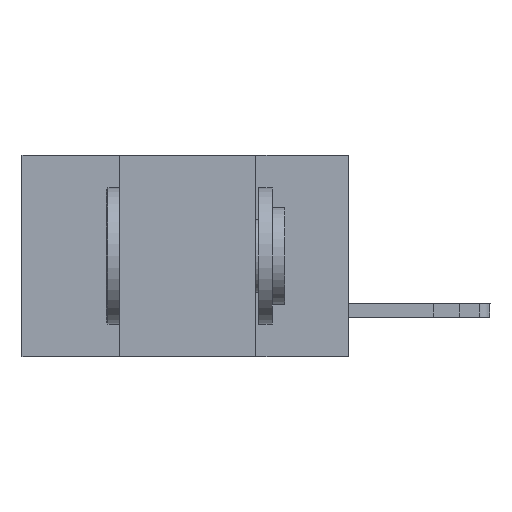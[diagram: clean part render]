
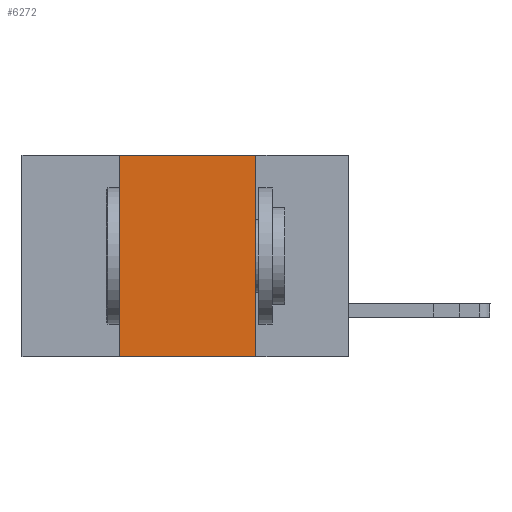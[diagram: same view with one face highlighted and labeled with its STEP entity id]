
A CAD part, left-side view. The second image highlights one B-rep face of the part: STEP entity #6272.
In plain terms, the highlighted planar face has unit normal (-1, 0, 0).
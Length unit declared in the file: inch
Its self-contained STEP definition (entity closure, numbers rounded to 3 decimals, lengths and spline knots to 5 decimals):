
#398 = VERTEX_POINT ( 'NONE', #16084 ) ;
#685 = ORIENTED_EDGE ( 'NONE', *, *, #16690, .F. ) ;
#1349 = EDGE_CURVE ( 'NONE', #14114, #12166, #11233, .T. ) ;
#2621 = CARTESIAN_POINT ( 'NONE',  ( 0., 0.42, -0.37 ) ) ;
#2738 = VECTOR ( 'NONE', #12178, 39.37008 ) ;
#2778 = CARTESIAN_POINT ( 'NONE',  ( 0., 0.6, -0.37 ) ) ;
#3225 = ORIENTED_EDGE ( 'NONE', *, *, #12811, .T. ) ;
#3415 = DIRECTION ( 'NONE',  ( 1., 0., 0. ) ) ;
#4107 = VERTEX_POINT ( 'NONE', #16202 ) ;
#4130 = DIRECTION ( 'NONE',  ( 0., 0., 1. ) ) ;
#5352 = LINE ( 'NONE', #6187, #16735 ) ;
#6187 = CARTESIAN_POINT ( 'NONE',  ( 0., 0.6, 0. ) ) ;
#6272 = ADVANCED_FACE ( 'NONE', ( #17154 ), #11888, .F. ) ;
#6337 = VECTOR ( 'NONE', #4130, 39.37008 ) ;
#6991 = CARTESIAN_POINT ( 'NONE',  ( 0., 0.6, 0. ) ) ;
#7690 = DIRECTION ( 'NONE',  ( 0., 0., -1. ) ) ;
#7740 = AXIS2_PLACEMENT_3D ( 'NONE', #6991, #3415, #7690 ) ;
#9054 = EDGE_LOOP ( 'NONE', ( #10799, #685, #9604, #3225 ) ) ;
#9604 = ORIENTED_EDGE ( 'NONE', *, *, #15727, .F. ) ;
#10799 = ORIENTED_EDGE ( 'NONE', *, *, #1349, .F. ) ;
#11233 = LINE ( 'NONE', #11684, #2738 ) ;
#11528 = LINE ( 'NONE', #2778, #12010 ) ;
#11684 = CARTESIAN_POINT ( 'NONE',  ( 0., 0.17, -0.37 ) ) ;
#11888 = PLANE ( 'NONE',  #7740 ) ;
#12010 = VECTOR ( 'NONE', #14726, 39.37008 ) ;
#12166 = VERTEX_POINT ( 'NONE', #18737 ) ;
#12178 = DIRECTION ( 'NONE',  ( 0., 0., -1. ) ) ;
#12665 = CARTESIAN_POINT ( 'NONE',  ( 0., 0.17, 0. ) ) ;
#12811 = EDGE_CURVE ( 'NONE', #4107, #12166, #11528, .T. ) ;
#14114 = VERTEX_POINT ( 'NONE', #12665 ) ;
#14726 = DIRECTION ( 'NONE',  ( 0., -1., 0. ) ) ;
#15727 = EDGE_CURVE ( 'NONE', #4107, #398, #18097, .T. ) ;
#16084 = CARTESIAN_POINT ( 'NONE',  ( 0., 0.42, 0. ) ) ;
#16202 = CARTESIAN_POINT ( 'NONE',  ( 0., 0.42, -0.37 ) ) ;
#16690 = EDGE_CURVE ( 'NONE', #398, #14114, #5352, .T. ) ;
#16735 = VECTOR ( 'NONE', #18805, 39.37008 ) ;
#17154 = FACE_OUTER_BOUND ( 'NONE', #9054, .T. ) ;
#18097 = LINE ( 'NONE', #2621, #6337 ) ;
#18737 = CARTESIAN_POINT ( 'NONE',  ( 0., 0.17, -0.37 ) ) ;
#18805 = DIRECTION ( 'NONE',  ( 0., -1., 0. ) ) ;
